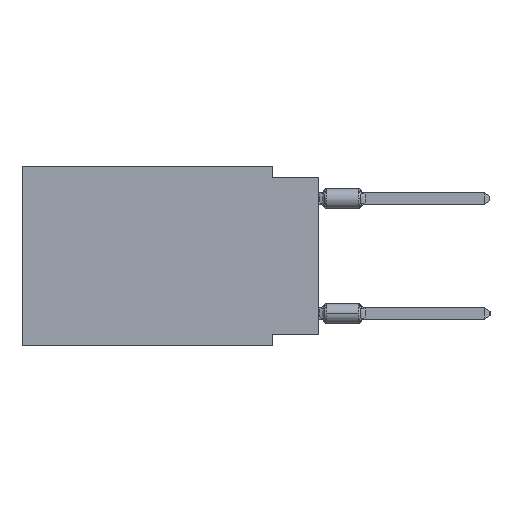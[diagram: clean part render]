
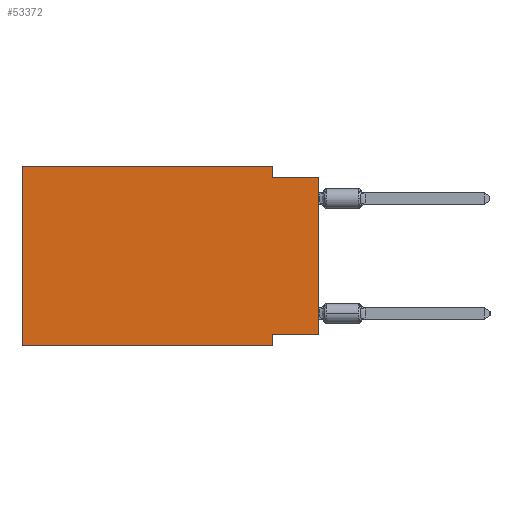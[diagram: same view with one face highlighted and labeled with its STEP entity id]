
A CAD part, left-side view. The second image highlights one B-rep face of the part: STEP entity #53372.
In plain terms, the highlighted planar face has unit normal (-1, 0, 0).
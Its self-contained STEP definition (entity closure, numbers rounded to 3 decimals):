
#2180 = AXIS2_PLACEMENT_3D ( 'NONE', #35886, #25233, #21767 ) ;
#2347 = DIRECTION ( 'NONE',  ( 0., 0., -1. ) ) ;
#4709 = CARTESIAN_POINT ( 'NONE',  ( 0., 2.54, -0.635 ) ) ;
#6961 = LINE ( 'NONE', #53763, #44922 ) ;
#7300 = DIRECTION ( 'NONE',  ( 0., 0., 1. ) ) ;
#7315 = PLANE ( 'NONE',  #2180 ) ;
#7805 = VERTEX_POINT ( 'NONE', #13371 ) ;
#9194 = VECTOR ( 'NONE', #29342, 1000. ) ;
#9576 = VERTEX_POINT ( 'NONE', #33974 ) ;
#9862 = VERTEX_POINT ( 'NONE', #53382 ) ;
#10480 = VERTEX_POINT ( 'NONE', #16233 ) ;
#12366 = VECTOR ( 'NONE', #39550, 1000. ) ;
#13371 = CARTESIAN_POINT ( 'NONE',  ( 0., 0., -9.271 ) ) ;
#14580 = ORIENTED_EDGE ( 'NONE', *, *, #31669, .F. ) ;
#15448 = DIRECTION ( 'NONE',  ( 0., 0., -1. ) ) ;
#15802 = VECTOR ( 'NONE', #2347, 1000. ) ;
#15849 = CARTESIAN_POINT ( 'NONE',  ( 0., 2.54, -9.906 ) ) ;
#16233 = CARTESIAN_POINT ( 'NONE',  ( 0., 16.383, 0. ) ) ;
#17564 = VERTEX_POINT ( 'NONE', #18555 ) ;
#18510 = LINE ( 'NONE', #32333, #39623 ) ;
#18555 = CARTESIAN_POINT ( 'NONE',  ( 0., 2.54, -9.271 ) ) ;
#18652 = ORIENTED_EDGE ( 'NONE', *, *, #34456, .F. ) ;
#19380 = ORIENTED_EDGE ( 'NONE', *, *, #42783, .T. ) ;
#19781 = CARTESIAN_POINT ( 'NONE',  ( 0., 0., -9.271 ) ) ;
#20216 = VERTEX_POINT ( 'NONE', #21893 ) ;
#20433 = CARTESIAN_POINT ( 'NONE',  ( 0., 16.383, 0. ) ) ;
#21767 = DIRECTION ( 'NONE',  ( 0., 0., -1. ) ) ;
#21893 = CARTESIAN_POINT ( 'NONE',  ( 0., 2.54, 0. ) ) ;
#23926 = ORIENTED_EDGE ( 'NONE', *, *, #56737, .F. ) ;
#24011 = LINE ( 'NONE', #48783, #9194 ) ;
#25233 = DIRECTION ( 'NONE',  ( 1., 0., 0. ) ) ;
#25433 = LINE ( 'NONE', #20433, #12366 ) ;
#28129 = VERTEX_POINT ( 'NONE', #29204 ) ;
#29204 = CARTESIAN_POINT ( 'NONE',  ( 0., 16.383, -9.906 ) ) ;
#29342 = DIRECTION ( 'NONE',  ( 0., -1., 0. ) ) ;
#31669 = EDGE_CURVE ( 'NONE', #7805, #17564, #53050, .T. ) ;
#32333 = CARTESIAN_POINT ( 'NONE',  ( 0., 0., -0.635 ) ) ;
#32937 = DIRECTION ( 'NONE',  ( 0., -1., 0. ) ) ;
#33301 = DIRECTION ( 'NONE',  ( 0., 1., 0. ) ) ;
#33974 = CARTESIAN_POINT ( 'NONE',  ( 0., 2.54, -9.906 ) ) ;
#34456 = EDGE_CURVE ( 'NONE', #45606, #9862, #18510, .T. ) ;
#34593 = CARTESIAN_POINT ( 'NONE',  ( 0., 2.54, 0. ) ) ;
#35511 = LINE ( 'NONE', #34593, #47706 ) ;
#35886 = CARTESIAN_POINT ( 'NONE',  ( 0., 16.383, 0. ) ) ;
#37423 = EDGE_CURVE ( 'NONE', #17564, #9576, #54756, .T. ) ;
#37844 = EDGE_CURVE ( 'NONE', #28129, #10480, #6961, .T. ) ;
#39550 = DIRECTION ( 'NONE',  ( 0., -1., 0. ) ) ;
#39623 = VECTOR ( 'NONE', #32937, 1000. ) ;
#40257 = LINE ( 'NONE', #46240, #53199 ) ;
#42783 = EDGE_CURVE ( 'NONE', #7805, #9862, #40257, .T. ) ;
#44054 = VECTOR ( 'NONE', #33301, 1000. ) ;
#44922 = VECTOR ( 'NONE', #58745, 1000. ) ;
#45384 = ORIENTED_EDGE ( 'NONE', *, *, #37423, .F. ) ;
#45606 = VERTEX_POINT ( 'NONE', #4709 ) ;
#46240 = CARTESIAN_POINT ( 'NONE',  ( 0., 0., 0. ) ) ;
#47294 = ORIENTED_EDGE ( 'NONE', *, *, #59856, .F. ) ;
#47706 = VECTOR ( 'NONE', #15448, 1000. ) ;
#48783 = CARTESIAN_POINT ( 'NONE',  ( 0., 16.383, -9.906 ) ) ;
#52580 = ORIENTED_EDGE ( 'NONE', *, *, #54561, .T. ) ;
#53050 = LINE ( 'NONE', #19781, #44054 ) ;
#53199 = VECTOR ( 'NONE', #7300, 1000. ) ;
#53372 = ADVANCED_FACE ( 'NONE', ( #54409 ), #7315, .F. ) ;
#53382 = CARTESIAN_POINT ( 'NONE',  ( 0., 0., -0.635 ) ) ;
#53763 = CARTESIAN_POINT ( 'NONE',  ( 0., 16.383, 0. ) ) ;
#54278 = ORIENTED_EDGE ( 'NONE', *, *, #37844, .F. ) ;
#54409 = FACE_OUTER_BOUND ( 'NONE', #59158, .T. ) ;
#54561 = EDGE_CURVE ( 'NONE', #28129, #9576, #24011, .T. ) ;
#54756 = LINE ( 'NONE', #15849, #15802 ) ;
#56737 = EDGE_CURVE ( 'NONE', #10480, #20216, #25433, .T. ) ;
#58745 = DIRECTION ( 'NONE',  ( 0., 0., 1. ) ) ;
#59158 = EDGE_LOOP ( 'NONE', ( #19380, #18652, #47294, #23926, #54278, #52580, #45384, #14580 ) ) ;
#59856 = EDGE_CURVE ( 'NONE', #20216, #45606, #35511, .T. ) ;
